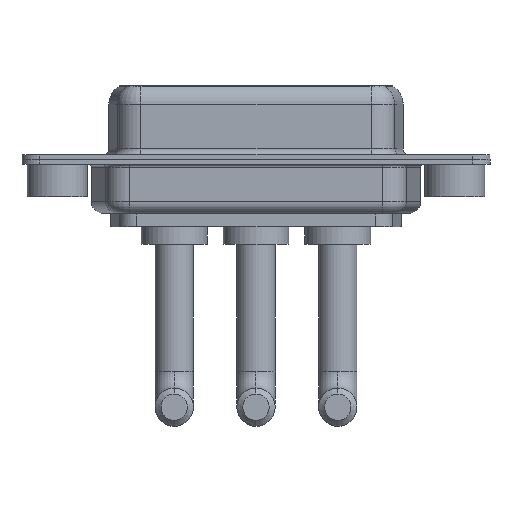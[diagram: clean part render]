
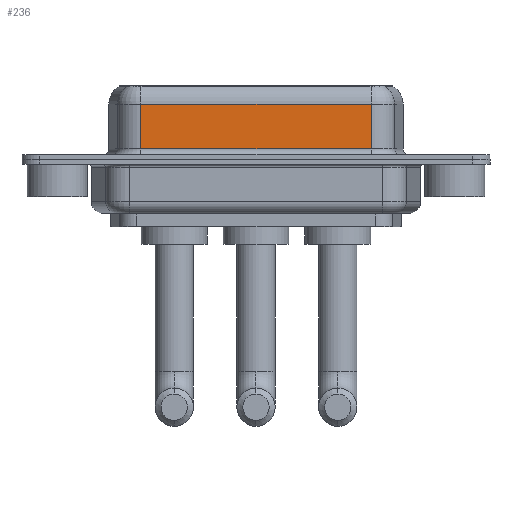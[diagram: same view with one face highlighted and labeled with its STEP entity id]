
A CAD part, front view. The second image highlights one B-rep face of the part: STEP entity #236.
In plain terms, the highlighted planar face has unit normal (0, -1, 0).
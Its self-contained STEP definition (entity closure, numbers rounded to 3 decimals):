
#28 = VECTOR ( 'NONE', #2039, 1000. ) ;
#112 = VERTEX_POINT ( 'NONE', #3902 ) ;
#151 = CARTESIAN_POINT ( 'NONE',  ( 26.287, -3.95, 4.65 ) ) ;
#236 = ADVANCED_FACE ( 'NONE', ( #10091 ), #2465, .F. ) ;
#473 = LINE ( 'NONE', #9085, #11400 ) ;
#707 = DIRECTION ( 'NONE',  ( 0., 0., -1. ) ) ;
#2039 = DIRECTION ( 'NONE',  ( 0., 0., -1. ) ) ;
#2465 = PLANE ( 'NONE',  #3847 ) ;
#3282 = CARTESIAN_POINT ( 'NONE',  ( 7.013, -3.95, 6.4 ) ) ;
#3847 = AXIS2_PLACEMENT_3D ( 'NONE', #9208, #11383, #6618 ) ;
#3902 = CARTESIAN_POINT ( 'NONE',  ( 7.013, -3.95, 0.9 ) ) ;
#4318 = ORIENTED_EDGE ( 'NONE', *, *, #11259, .T. ) ;
#6233 = EDGE_CURVE ( 'NONE', #112, #8947, #473, .T. ) ;
#6461 = EDGE_CURVE ( 'NONE', #10111, #10211, #9493, .T. ) ;
#6618 = DIRECTION ( 'NONE',  ( 0., 0., 1. ) ) ;
#6732 = CARTESIAN_POINT ( 'NONE',  ( 7.013, -3.95, 4.65 ) ) ;
#7563 = DIRECTION ( 'NONE',  ( -1., 0., 0. ) ) ;
#7906 = CARTESIAN_POINT ( 'NONE',  ( 26.287, -3.95, 0.9 ) ) ;
#7950 = EDGE_LOOP ( 'NONE', ( #8319, #8637, #4318, #11487 ) ) ;
#8233 = EDGE_CURVE ( 'NONE', #10111, #8947, #9542, .T. ) ;
#8319 = ORIENTED_EDGE ( 'NONE', *, *, #8233, .F. ) ;
#8363 = VECTOR ( 'NONE', #7563, 1000. ) ;
#8637 = ORIENTED_EDGE ( 'NONE', *, *, #6461, .T. ) ;
#8904 = VECTOR ( 'NONE', #707, 1000. ) ;
#8947 = VERTEX_POINT ( 'NONE', #7906 ) ;
#9025 = DIRECTION ( 'NONE',  ( 1., 0., 0. ) ) ;
#9085 = CARTESIAN_POINT ( 'NONE',  ( 26.287, -3.95, 0.9 ) ) ;
#9157 = LINE ( 'NONE', #3282, #8904 ) ;
#9208 = CARTESIAN_POINT ( 'NONE',  ( 26.287, -3.95, 6.4 ) ) ;
#9430 = CARTESIAN_POINT ( 'NONE',  ( 26.287, -3.95, 4.65 ) ) ;
#9493 = LINE ( 'NONE', #9430, #8363 ) ;
#9542 = LINE ( 'NONE', #10539, #28 ) ;
#10091 = FACE_OUTER_BOUND ( 'NONE', #7950, .T. ) ;
#10111 = VERTEX_POINT ( 'NONE', #151 ) ;
#10211 = VERTEX_POINT ( 'NONE', #6732 ) ;
#10539 = CARTESIAN_POINT ( 'NONE',  ( 26.287, -3.95, 6.4 ) ) ;
#11259 = EDGE_CURVE ( 'NONE', #10211, #112, #9157, .T. ) ;
#11383 = DIRECTION ( 'NONE',  ( 0., 1., 0. ) ) ;
#11400 = VECTOR ( 'NONE', #9025, 1000. ) ;
#11487 = ORIENTED_EDGE ( 'NONE', *, *, #6233, .T. ) ;
